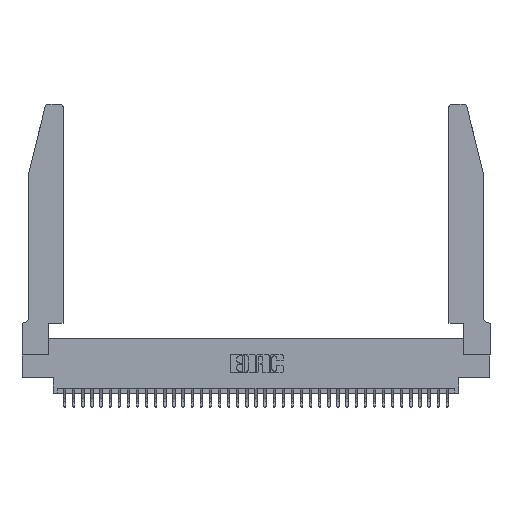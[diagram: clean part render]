
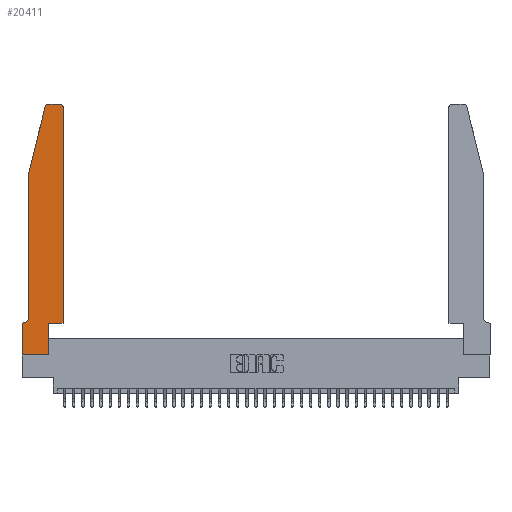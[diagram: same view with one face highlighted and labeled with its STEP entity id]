
A CAD part, top view. The second image highlights one B-rep face of the part: STEP entity #20411.
In plain terms, the highlighted planar face has unit normal (0, 0, 1).
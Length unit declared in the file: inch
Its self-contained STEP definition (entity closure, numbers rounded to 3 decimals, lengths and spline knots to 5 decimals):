
#17 = VECTOR ( 'NONE', #18588, 39.37008 ) ;
#133 = VERTEX_POINT ( 'NONE', #13185 ) ;
#1553 = DIRECTION ( 'NONE',  ( 1., 0., 0. ) ) ;
#1865 = ORIENTED_EDGE ( 'NONE', *, *, #11077, .T. ) ;
#1877 = VECTOR ( 'NONE', #6340, 39.37008 ) ;
#2933 = VECTOR ( 'NONE', #34918, 39.37008 ) ;
#3510 = LINE ( 'NONE', #30760, #11503 ) ;
#3755 = EDGE_CURVE ( 'NONE', #36334, #29793, #19779, .T. ) ;
#3937 = VERTEX_POINT ( 'NONE', #7380 ) ;
#4045 = VECTOR ( 'NONE', #14015, 39.37008 ) ;
#4689 = CIRCLE ( 'NONE', #16411, 0.07 ) ;
#4828 = PLANE ( 'NONE',  #5867 ) ;
#5416 = ORIENTED_EDGE ( 'NONE', *, *, #29266, .T. ) ;
#5591 = CARTESIAN_POINT ( 'NONE',  ( 0.0755, 2., 0.37 ) ) ;
#5867 = AXIS2_PLACEMENT_3D ( 'NONE', #7833, #31373, #1553 ) ;
#5882 = DIRECTION ( 'NONE',  ( 0., 0., -1. ) ) ;
#6191 = VERTEX_POINT ( 'NONE', #29929 ) ;
#6340 = DIRECTION ( 'NONE',  ( 0., -1., 0. ) ) ;
#6600 = FACE_OUTER_BOUND ( 'NONE', #9458, .T. ) ;
#6612 = DIRECTION ( 'NONE',  ( 1., 0., 0. ) ) ;
#7003 = LINE ( 'NONE', #30165, #13998 ) ;
#7380 = CARTESIAN_POINT ( 'NONE',  ( 0.0755, 2., 0.37 ) ) ;
#7833 = CARTESIAN_POINT ( 'NONE',  ( 0., 0.35, 0.37 ) ) ;
#7880 = ORIENTED_EDGE ( 'NONE', *, *, #21180, .T. ) ;
#7976 = LINE ( 'NONE', #5591, #17 ) ;
#8024 = ORIENTED_EDGE ( 'NONE', *, *, #21419, .T. ) ;
#8324 = CARTESIAN_POINT ( 'NONE',  ( 0.0755, 2., 0.37 ) ) ;
#8893 = LINE ( 'NONE', #35738, #29476 ) ;
#8913 = CARTESIAN_POINT ( 'NONE',  ( 0.0055, 0.42, 0.37 ) ) ;
#9311 = ORIENTED_EDGE ( 'NONE', *, *, #3755, .T. ) ;
#9458 = EDGE_LOOP ( 'NONE', ( #34227, #31731, #7880, #35014, #37183, #9311, #13915, #8024, #18275, #1865, #29994, #5416 ) ) ;
#9764 = VERTEX_POINT ( 'NONE', #15976 ) ;
#10164 = DIRECTION ( 'NONE',  ( 1., 0., 0. ) ) ;
#11064 = EDGE_CURVE ( 'NONE', #14372, #16108, #23445, .T. ) ;
#11077 = EDGE_CURVE ( 'NONE', #6191, #14826, #7003, .T. ) ;
#11210 = DIRECTION ( 'NONE',  ( -0.239, -0.971, 0. ) ) ;
#11503 = VECTOR ( 'NONE', #15866, 39.37008 ) ;
#12015 = CIRCLE ( 'NONE', #19099, 0.03 ) ;
#12371 = VERTEX_POINT ( 'NONE', #30651 ) ;
#12468 = EDGE_CURVE ( 'NONE', #3937, #33845, #7976, .T. ) ;
#13087 = CARTESIAN_POINT ( 'NONE',  ( 0.0755, 0.42, 0.37 ) ) ;
#13185 = CARTESIAN_POINT ( 'NONE',  ( 0., 0., 0.37 ) ) ;
#13915 = ORIENTED_EDGE ( 'NONE', *, *, #38374, .T. ) ;
#13998 = VECTOR ( 'NONE', #6612, 39.37008 ) ;
#14015 = DIRECTION ( 'NONE',  ( 0., 1., 0. ) ) ;
#14372 = VERTEX_POINT ( 'NONE', #15796 ) ;
#14826 = VERTEX_POINT ( 'NONE', #26374 ) ;
#15413 = EDGE_CURVE ( 'NONE', #12371, #6191, #3510, .T. ) ;
#15466 = LINE ( 'NONE', #33361, #1877 ) ;
#15796 = CARTESIAN_POINT ( 'NONE',  ( 0.284, 2.75, 0.37 ) ) ;
#15861 = DIRECTION ( 'NONE',  ( -1., 0., 0. ) ) ;
#15866 = DIRECTION ( 'NONE',  ( 0., 1., 0. ) ) ;
#15976 = CARTESIAN_POINT ( 'NONE',  ( 0.4205, 2.75, 0.37 ) ) ;
#16108 = VERTEX_POINT ( 'NONE', #37192 ) ;
#16411 = AXIS2_PLACEMENT_3D ( 'NONE', #8913, #5882, #35527 ) ;
#17761 = CARTESIAN_POINT ( 'NONE',  ( 0.2605, 2.75, 0.37 ) ) ;
#18157 = LINE ( 'NONE', #17761, #27993 ) ;
#18275 = ORIENTED_EDGE ( 'NONE', *, *, #15413, .T. ) ;
#18588 = DIRECTION ( 'NONE',  ( 0., -1., 0. ) ) ;
#19099 = AXIS2_PLACEMENT_3D ( 'NONE', #25904, #31666, #22618 ) ;
#19509 = LINE ( 'NONE', #29050, #4045 ) ;
#19779 = LINE ( 'NONE', #22640, #2933 ) ;
#20141 = AXIS2_PLACEMENT_3D ( 'NONE', #33768, #30923, #10164 ) ;
#20411 = ADVANCED_FACE ( 'NONE', ( #6600 ), #4828, .T. ) ;
#20879 = CARTESIAN_POINT ( 'NONE',  ( 0.0055, 0.35, 0.37 ) ) ;
#21180 = EDGE_CURVE ( 'NONE', #16108, #3937, #31328, .T. ) ;
#21419 = EDGE_CURVE ( 'NONE', #133, #12371, #8893, .T. ) ;
#22618 = DIRECTION ( 'NONE',  ( 1., 0., 0. ) ) ;
#22640 = CARTESIAN_POINT ( 'NONE',  ( 0.0755, 0.35, 0.37 ) ) ;
#22702 = EDGE_CURVE ( 'NONE', #9764, #14372, #18157, .T. ) ;
#23445 = CIRCLE ( 'NONE', #20141, 0.03 ) ;
#23859 = VECTOR ( 'NONE', #11210, 39.37008 ) ;
#23991 = VERTEX_POINT ( 'NONE', #33649 ) ;
#25904 = CARTESIAN_POINT ( 'NONE',  ( 0.4205, 2.72, 0.37 ) ) ;
#26374 = CARTESIAN_POINT ( 'NONE',  ( 0.4505, 0.35, 0.37 ) ) ;
#27993 = VECTOR ( 'NONE', #15861, 39.37008 ) ;
#29050 = CARTESIAN_POINT ( 'NONE',  ( 0.4505, 0.35, 0.37 ) ) ;
#29201 = EDGE_CURVE ( 'NONE', #14826, #23991, #19509, .T. ) ;
#29266 = EDGE_CURVE ( 'NONE', #23991, #9764, #12015, .T. ) ;
#29476 = VECTOR ( 'NONE', #35991, 39.37008 ) ;
#29793 = VERTEX_POINT ( 'NONE', #37459 ) ;
#29929 = CARTESIAN_POINT ( 'NONE',  ( 0.2865, 0.35, 0.37 ) ) ;
#29994 = ORIENTED_EDGE ( 'NONE', *, *, #29201, .T. ) ;
#30165 = CARTESIAN_POINT ( 'NONE',  ( 0.4505, 0.35, 0.37 ) ) ;
#30651 = CARTESIAN_POINT ( 'NONE',  ( 0.2865, 0., 0.37 ) ) ;
#30760 = CARTESIAN_POINT ( 'NONE',  ( 0.2865, 0.35, 0.37 ) ) ;
#30923 = DIRECTION ( 'NONE',  ( 0., 0., 1. ) ) ;
#31328 = LINE ( 'NONE', #8324, #23859 ) ;
#31373 = DIRECTION ( 'NONE',  ( 0., 0., 1. ) ) ;
#31666 = DIRECTION ( 'NONE',  ( 0., 0., 1. ) ) ;
#31731 = ORIENTED_EDGE ( 'NONE', *, *, #11064, .T. ) ;
#33361 = CARTESIAN_POINT ( 'NONE',  ( 0., 0., 0.37 ) ) ;
#33649 = CARTESIAN_POINT ( 'NONE',  ( 0.4505, 2.72, 0.37 ) ) ;
#33768 = CARTESIAN_POINT ( 'NONE',  ( 0.284, 2.72, 0.37 ) ) ;
#33845 = VERTEX_POINT ( 'NONE', #13087 ) ;
#34227 = ORIENTED_EDGE ( 'NONE', *, *, #22702, .T. ) ;
#34320 = EDGE_CURVE ( 'NONE', #33845, #36334, #4689, .T. ) ;
#34918 = DIRECTION ( 'NONE',  ( -1., 0., 0. ) ) ;
#35014 = ORIENTED_EDGE ( 'NONE', *, *, #12468, .T. ) ;
#35527 = DIRECTION ( 'NONE',  ( -1., 0., 0. ) ) ;
#35738 = CARTESIAN_POINT ( 'NONE',  ( 0., 0., 0.37 ) ) ;
#35991 = DIRECTION ( 'NONE',  ( 1., 0., 0. ) ) ;
#36334 = VERTEX_POINT ( 'NONE', #20879 ) ;
#37183 = ORIENTED_EDGE ( 'NONE', *, *, #34320, .T. ) ;
#37192 = CARTESIAN_POINT ( 'NONE',  ( 0.25487, 2.72718, 0.37 ) ) ;
#37459 = CARTESIAN_POINT ( 'NONE',  ( 0., 0.35, 0.37 ) ) ;
#38374 = EDGE_CURVE ( 'NONE', #29793, #133, #15466, .T. ) ;
